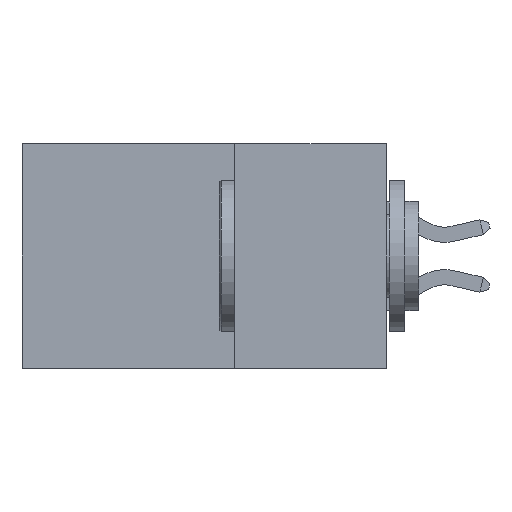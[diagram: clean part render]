
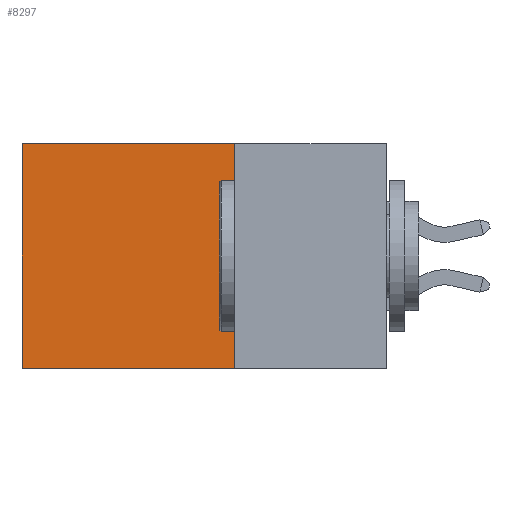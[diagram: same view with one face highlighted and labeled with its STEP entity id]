
A CAD part, left-side view. The second image highlights one B-rep face of the part: STEP entity #8297.
In plain terms, the highlighted planar face has unit normal (-1, 0, 0).
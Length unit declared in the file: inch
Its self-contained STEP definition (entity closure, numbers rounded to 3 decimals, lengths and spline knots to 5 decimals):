
#849 = DIRECTION ( 'NONE',  ( 0., 1., 0. ) ) ;
#1139 = CARTESIAN_POINT ( 'NONE',  ( 0.298, 0.25, 0. ) ) ;
#1164 = VECTOR ( 'NONE', #4902, 39.37008 ) ;
#1599 = LINE ( 'NONE', #2769, #5430 ) ;
#1983 = DIRECTION ( 'NONE',  ( 0., 1., 0. ) ) ;
#2769 = CARTESIAN_POINT ( 'NONE',  ( 0.298, 0.25, 0. ) ) ;
#2887 = LINE ( 'NONE', #19864, #15104 ) ;
#3386 = ORIENTED_EDGE ( 'NONE', *, *, #8065, .F. ) ;
#3882 = VERTEX_POINT ( 'NONE', #7880 ) ;
#4902 = DIRECTION ( 'NONE',  ( 0., 0., -1. ) ) ;
#5430 = VECTOR ( 'NONE', #15522, 39.37008 ) ;
#6408 = PLANE ( 'NONE',  #9466 ) ;
#6472 = VECTOR ( 'NONE', #1983, 39.37008 ) ;
#7500 = LINE ( 'NONE', #19325, #6472 ) ;
#7880 = CARTESIAN_POINT ( 'NONE',  ( 0.298, 0.25, -0.37 ) ) ;
#7984 = VERTEX_POINT ( 'NONE', #8929 ) ;
#8033 = DIRECTION ( 'NONE',  ( 1., 0., 0. ) ) ;
#8065 = EDGE_CURVE ( 'NONE', #19321, #3882, #1599, .T. ) ;
#8297 = ADVANCED_FACE ( 'NONE', ( #19717 ), #6408, .F. ) ;
#8929 = CARTESIAN_POINT ( 'NONE',  ( 0.298, 0.6, -0.37 ) ) ;
#9301 = ORIENTED_EDGE ( 'NONE', *, *, #11309, .F. ) ;
#9466 = AXIS2_PLACEMENT_3D ( 'NONE', #11143, #8033, #19025 ) ;
#9823 = EDGE_CURVE ( 'NONE', #15780, #7984, #13498, .T. ) ;
#11143 = CARTESIAN_POINT ( 'NONE',  ( 0.298, 0.25, 0. ) ) ;
#11229 = CARTESIAN_POINT ( 'NONE',  ( 0.298, 0.6, 0. ) ) ;
#11309 = EDGE_CURVE ( 'NONE', #3882, #7984, #7500, .T. ) ;
#12351 = EDGE_LOOP ( 'NONE', ( #19201, #9301, #3386, #18814 ) ) ;
#13498 = LINE ( 'NONE', #11229, #1164 ) ;
#14487 = CARTESIAN_POINT ( 'NONE',  ( 0.298, 0.6, 0. ) ) ;
#15104 = VECTOR ( 'NONE', #849, 39.37008 ) ;
#15355 = EDGE_CURVE ( 'NONE', #19321, #15780, #2887, .T. ) ;
#15522 = DIRECTION ( 'NONE',  ( 0., 0., -1. ) ) ;
#15780 = VERTEX_POINT ( 'NONE', #14487 ) ;
#18814 = ORIENTED_EDGE ( 'NONE', *, *, #15355, .T. ) ;
#19025 = DIRECTION ( 'NONE',  ( 0., 0., -1. ) ) ;
#19201 = ORIENTED_EDGE ( 'NONE', *, *, #9823, .T. ) ;
#19321 = VERTEX_POINT ( 'NONE', #1139 ) ;
#19325 = CARTESIAN_POINT ( 'NONE',  ( 0.298, 0.25, -0.37 ) ) ;
#19717 = FACE_OUTER_BOUND ( 'NONE', #12351, .T. ) ;
#19864 = CARTESIAN_POINT ( 'NONE',  ( 0.298, 0.25, 0. ) ) ;
